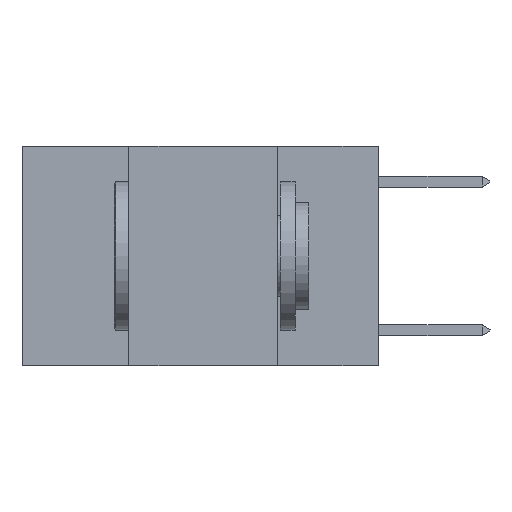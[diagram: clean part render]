
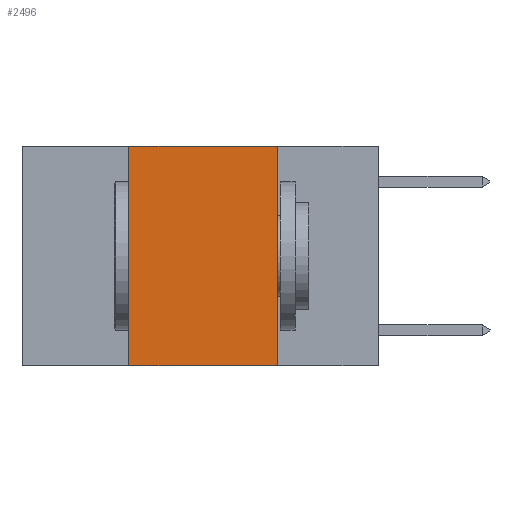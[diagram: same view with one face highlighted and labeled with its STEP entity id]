
A CAD part, left-side view. The second image highlights one B-rep face of the part: STEP entity #2496.
In plain terms, the highlighted planar face has unit normal (-1, 0, 0).
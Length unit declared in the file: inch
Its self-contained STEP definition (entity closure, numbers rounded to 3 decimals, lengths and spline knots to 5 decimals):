
#176 = CARTESIAN_POINT ( 'NONE',  ( 0., 0.17, 0. ) ) ;
#505 = LINE ( 'NONE', #5268, #22690 ) ;
#808 = VERTEX_POINT ( 'NONE', #7295 ) ;
#1024 = DIRECTION ( 'NONE',  ( 0., 0., 1. ) ) ;
#2496 = ADVANCED_FACE ( 'NONE', ( #18994 ), #21596, .F. ) ;
#2586 = CARTESIAN_POINT ( 'NONE',  ( 0., 0.6, 0. ) ) ;
#4264 = ORIENTED_EDGE ( 'NONE', *, *, #6851, .F. ) ;
#4414 = ORIENTED_EDGE ( 'NONE', *, *, #21974, .F. ) ;
#5268 = CARTESIAN_POINT ( 'NONE',  ( 0., 0.42, 0. ) ) ;
#5453 = DIRECTION ( 'NONE',  ( 0., -1., 0. ) ) ;
#5578 = LINE ( 'NONE', #2586, #16798 ) ;
#5719 = AXIS2_PLACEMENT_3D ( 'NONE', #11335, #25611, #13406 ) ;
#6403 = EDGE_LOOP ( 'NONE', ( #4264, #4414, #7283, #16281 ) ) ;
#6851 = EDGE_CURVE ( 'NONE', #20548, #25437, #15414, .T. ) ;
#7283 = ORIENTED_EDGE ( 'NONE', *, *, #17476, .F. ) ;
#7295 = CARTESIAN_POINT ( 'NONE',  ( 0., 0.42, 0. ) ) ;
#7439 = CARTESIAN_POINT ( 'NONE',  ( 0., 0.17, 0. ) ) ;
#9582 = DIRECTION ( 'NONE',  ( 0., 0., -1. ) ) ;
#11335 = CARTESIAN_POINT ( 'NONE',  ( 0., 0.6, 0. ) ) ;
#12115 = CARTESIAN_POINT ( 'NONE',  ( 0., 0.17, -0.37 ) ) ;
#12590 = CARTESIAN_POINT ( 'NONE',  ( 0., 0.42, -0.37 ) ) ;
#13406 = DIRECTION ( 'NONE',  ( 0., 0., -1. ) ) ;
#15253 = DIRECTION ( 'NONE',  ( 0., -1., 0. ) ) ;
#15313 = VECTOR ( 'NONE', #9582, 39.37008 ) ;
#15393 = LINE ( 'NONE', #26122, #17973 ) ;
#15414 = LINE ( 'NONE', #7439, #15313 ) ;
#16281 = ORIENTED_EDGE ( 'NONE', *, *, #17552, .T. ) ;
#16798 = VECTOR ( 'NONE', #15253, 39.37008 ) ;
#17476 = EDGE_CURVE ( 'NONE', #24375, #808, #505, .T. ) ;
#17552 = EDGE_CURVE ( 'NONE', #24375, #25437, #15393, .T. ) ;
#17973 = VECTOR ( 'NONE', #5453, 39.37008 ) ;
#18994 = FACE_OUTER_BOUND ( 'NONE', #6403, .T. ) ;
#20548 = VERTEX_POINT ( 'NONE', #176 ) ;
#21596 = PLANE ( 'NONE',  #5719 ) ;
#21974 = EDGE_CURVE ( 'NONE', #808, #20548, #5578, .T. ) ;
#22690 = VECTOR ( 'NONE', #1024, 39.37008 ) ;
#24375 = VERTEX_POINT ( 'NONE', #12590 ) ;
#25437 = VERTEX_POINT ( 'NONE', #12115 ) ;
#25611 = DIRECTION ( 'NONE',  ( 1., 0., 0. ) ) ;
#26122 = CARTESIAN_POINT ( 'NONE',  ( 0., 0.6, -0.37 ) ) ;
